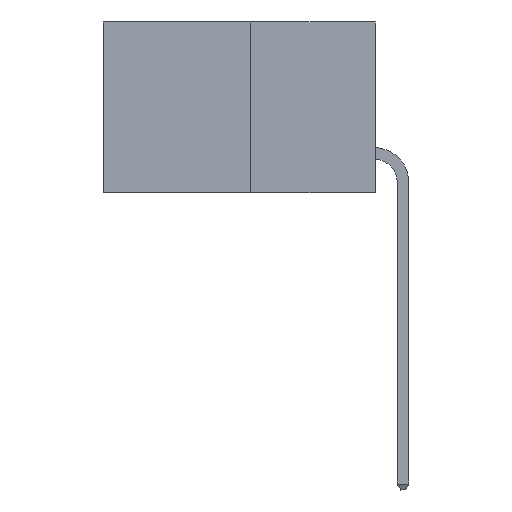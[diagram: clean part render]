
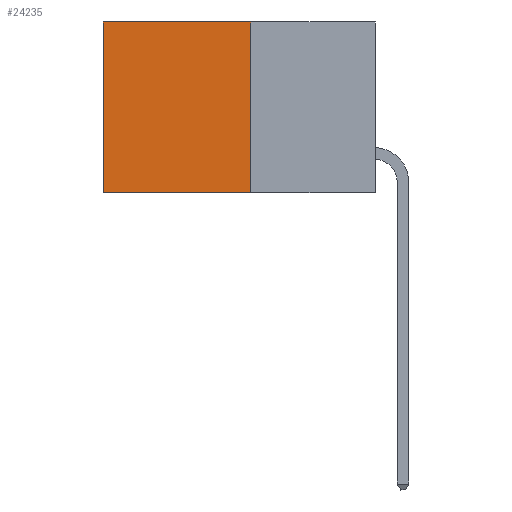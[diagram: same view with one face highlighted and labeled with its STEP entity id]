
A CAD part, left-side view. The second image highlights one B-rep face of the part: STEP entity #24235.
In plain terms, the highlighted planar face has unit normal (-1, 0, 0).
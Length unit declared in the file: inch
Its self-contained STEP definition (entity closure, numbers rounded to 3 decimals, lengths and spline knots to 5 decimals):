
#832 = LINE ( 'NONE', #11770, #10281 ) ;
#1124 = CARTESIAN_POINT ( 'NONE',  ( 0.277, 0.27, -0.37 ) ) ;
#1308 = ORIENTED_EDGE ( 'NONE', *, *, #20951, .T. ) ;
#1743 = CARTESIAN_POINT ( 'NONE',  ( 0.277, 0.59, 0. ) ) ;
#2885 = VERTEX_POINT ( 'NONE', #21956 ) ;
#3233 = ORIENTED_EDGE ( 'NONE', *, *, #6992, .T. ) ;
#4063 = LINE ( 'NONE', #10264, #7884 ) ;
#4155 = LINE ( 'NONE', #19475, #22351 ) ;
#4726 = CARTESIAN_POINT ( 'NONE',  ( 0.277, 0.27, -0.37 ) ) ;
#6101 = FACE_OUTER_BOUND ( 'NONE', #6993, .T. ) ;
#6599 = DIRECTION ( 'NONE',  ( 1., 0., 0. ) ) ;
#6992 = EDGE_CURVE ( 'NONE', #2885, #22531, #4063, .T. ) ;
#6993 = EDGE_LOOP ( 'NONE', ( #1308, #15269, #21116, #3233 ) ) ;
#7884 = VECTOR ( 'NONE', #21458, 39.37008 ) ;
#10264 = CARTESIAN_POINT ( 'NONE',  ( 0.277, 0.27, 0. ) ) ;
#10281 = VECTOR ( 'NONE', #15505, 39.37008 ) ;
#10972 = CARTESIAN_POINT ( 'NONE',  ( 0.277, 0.59, -0.37 ) ) ;
#11770 = CARTESIAN_POINT ( 'NONE',  ( 0.277, 0.27, -0.37 ) ) ;
#11833 = EDGE_CURVE ( 'NONE', #20186, #15796, #832, .T. ) ;
#13575 = EDGE_CURVE ( 'NONE', #2885, #20186, #4155, .T. ) ;
#14863 = CARTESIAN_POINT ( 'NONE',  ( 0.277, 0.59, -0.37 ) ) ;
#15269 = ORIENTED_EDGE ( 'NONE', *, *, #11833, .F. ) ;
#15505 = DIRECTION ( 'NONE',  ( 0., 1., 0. ) ) ;
#15796 = VERTEX_POINT ( 'NONE', #14863 ) ;
#17654 = AXIS2_PLACEMENT_3D ( 'NONE', #4726, #6599, #19718 ) ;
#17830 = PLANE ( 'NONE',  #17654 ) ;
#19475 = CARTESIAN_POINT ( 'NONE',  ( 0.277, 0.27, -0.37 ) ) ;
#19483 = LINE ( 'NONE', #10972, #23833 ) ;
#19718 = DIRECTION ( 'NONE',  ( 0., 0., -1. ) ) ;
#20186 = VERTEX_POINT ( 'NONE', #1124 ) ;
#20951 = EDGE_CURVE ( 'NONE', #22531, #15796, #19483, .T. ) ;
#21116 = ORIENTED_EDGE ( 'NONE', *, *, #13575, .F. ) ;
#21458 = DIRECTION ( 'NONE',  ( 0., 1., 0. ) ) ;
#21956 = CARTESIAN_POINT ( 'NONE',  ( 0.277, 0.27, 0. ) ) ;
#22198 = DIRECTION ( 'NONE',  ( 0., 0., -1. ) ) ;
#22351 = VECTOR ( 'NONE', #23149, 39.37008 ) ;
#22531 = VERTEX_POINT ( 'NONE', #1743 ) ;
#23149 = DIRECTION ( 'NONE',  ( 0., 0., -1. ) ) ;
#23833 = VECTOR ( 'NONE', #22198, 39.37008 ) ;
#24235 = ADVANCED_FACE ( 'NONE', ( #6101 ), #17830, .F. ) ;
